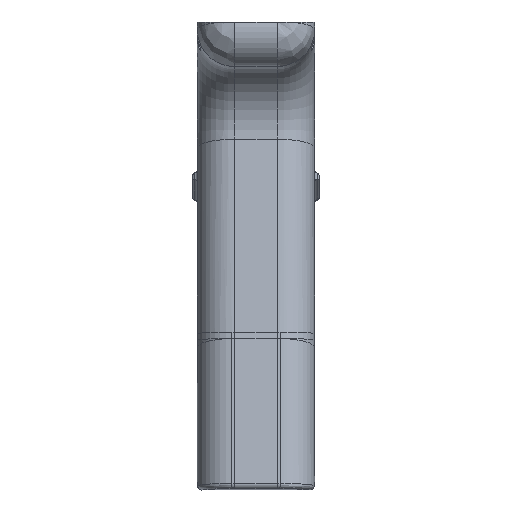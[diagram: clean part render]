
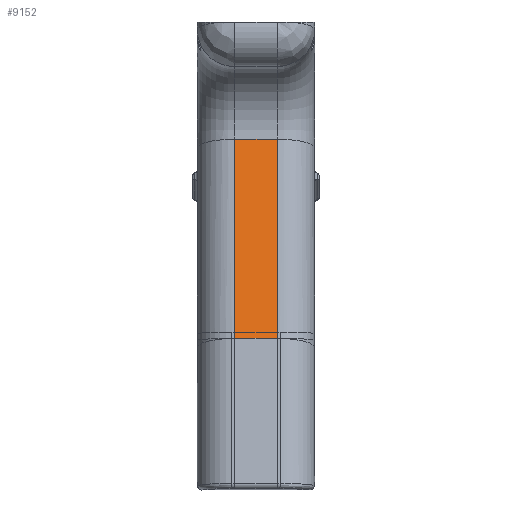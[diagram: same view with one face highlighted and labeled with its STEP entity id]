
A CAD part, front view. The second image highlights one B-rep face of the part: STEP entity #9152.
In plain terms, the highlighted face is planar.
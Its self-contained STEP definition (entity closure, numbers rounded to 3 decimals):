
#860=PLANE('',#9978);
#1270=FACE_OUTER_BOUND('',#1793,.T.);
#1793=EDGE_LOOP('',(#7898,#7899,#7900,#7901));
#2416=LINE('',#16182,#3174);
#2570=LINE('',#17027,#3328);
#2571=LINE('',#17030,#3329);
#2572=LINE('',#17031,#3330);
#3174=VECTOR('',#11675,10.);
#3328=VECTOR('',#12075,10.);
#3329=VECTOR('',#12078,10.);
#3330=VECTOR('',#12079,10.);
#4239=VERTEX_POINT('',#16178);
#4240=VERTEX_POINT('',#16180);
#4375=VERTEX_POINT('',#17005);
#4378=VERTEX_POINT('',#17029);
#5393=EDGE_CURVE('',#4239,#4240,#2416,.T.);
#5617=EDGE_CURVE('',#4239,#4375,#2570,.T.);
#5618=EDGE_CURVE('',#4378,#4240,#2571,.T.);
#5619=EDGE_CURVE('',#4375,#4378,#2572,.T.);
#7898=ORIENTED_EDGE('',*,*,#5618,.F.);
#7899=ORIENTED_EDGE('',*,*,#5619,.F.);
#7900=ORIENTED_EDGE('',*,*,#5617,.F.);
#7901=ORIENTED_EDGE('',*,*,#5393,.T.);
#9152=ADVANCED_FACE('',(#1270),#860,.T.);
#9978=AXIS2_PLACEMENT_3D('',#17028,#12076,#12077);
#11675=DIRECTION('',(0.,-0.249,0.969));
#12075=DIRECTION('',(-1.,0.,0.));
#12076=DIRECTION('center_axis',(0.,-0.969,
-0.249));
#12077=DIRECTION('ref_axis',(0.,-0.249,0.969));
#12078=DIRECTION('',(1.,0.,0.));
#12079=DIRECTION('',(0.,-0.249,0.969));
#16178=CARTESIAN_POINT('',(13.45,-71.634,19.877));
#16180=CARTESIAN_POINT('',(13.45,-83.628,66.536));
#16182=CARTESIAN_POINT('',(13.45,-83.554,66.245));
#17005=CARTESIAN_POINT('',(3.45,-71.634,19.877));
#17027=CARTESIAN_POINT('',(22.175,-71.634,19.877));
#17028=CARTESIAN_POINT('Origin',(22.175,-71.634,19.877));
#17029=CARTESIAN_POINT('',(3.45,-83.628,66.536));
#17030=CARTESIAN_POINT('',(22.175,-83.628,66.536));
#17031=CARTESIAN_POINT('',(3.45,-83.554,66.245));
